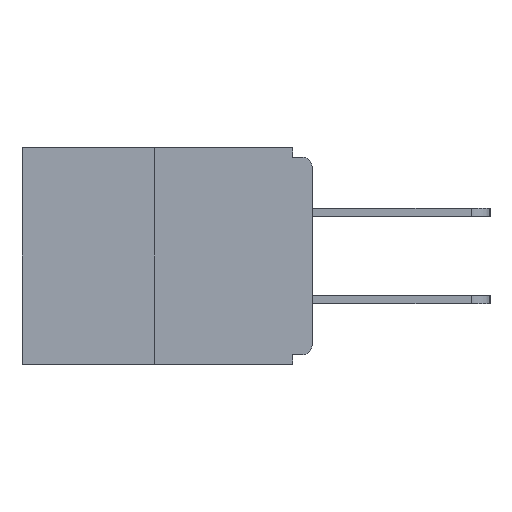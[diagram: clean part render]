
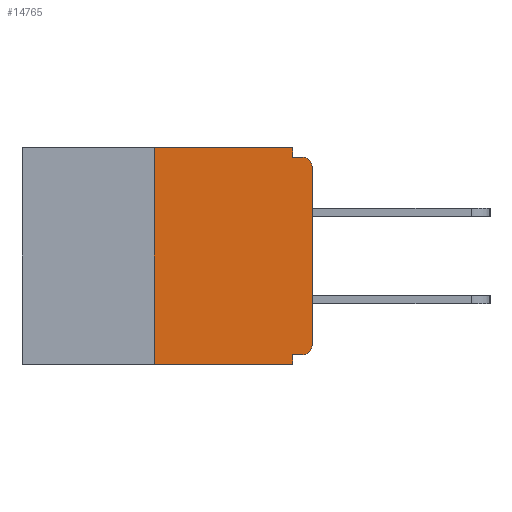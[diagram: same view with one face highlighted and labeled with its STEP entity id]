
A CAD part, left-side view. The second image highlights one B-rep face of the part: STEP entity #14765.
In plain terms, the highlighted planar face has unit normal (-1, 0, 0).
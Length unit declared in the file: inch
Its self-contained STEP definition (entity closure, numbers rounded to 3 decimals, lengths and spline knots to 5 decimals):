
#715 = DIRECTION ( 'NONE',  ( 0., 0., -1. ) ) ;
#1543 = CARTESIAN_POINT ( 'NONE',  ( 0., 0.015, -0.328 ) ) ;
#1964 = EDGE_CURVE ( 'NONE', #25171, #8974, #14584, .T. ) ;
#2256 = ORIENTED_EDGE ( 'NONE', *, *, #24477, .F. ) ;
#2329 = CARTESIAN_POINT ( 'NONE',  ( 0., 0.015, -0.03 ) ) ;
#2338 = VECTOR ( 'NONE', #20732, 39.37008 ) ;
#2395 = ORIENTED_EDGE ( 'NONE', *, *, #14337, .F. ) ;
#2488 = CARTESIAN_POINT ( 'NONE',  ( 0., 0.46, 0. ) ) ;
#2497 = VECTOR ( 'NONE', #12584, 39.37008 ) ;
#2853 = EDGE_CURVE ( 'NONE', #6195, #24756, #24557, .T. ) ;
#3083 = CIRCLE ( 'NONE', #25543, 0.015 ) ;
#3275 = ORIENTED_EDGE ( 'NONE', *, *, #10744, .T. ) ;
#3653 = VECTOR ( 'NONE', #22332, 39.37008 ) ;
#3779 = VECTOR ( 'NONE', #16435, 39.37008 ) ;
#3904 = DIRECTION ( 'NONE',  ( 0., 0., 1. ) ) ;
#4620 = CARTESIAN_POINT ( 'NONE',  ( 0., 0.031, -0.343 ) ) ;
#5089 = VECTOR ( 'NONE', #3904, 39.37008 ) ;
#6195 = VERTEX_POINT ( 'NONE', #13109 ) ;
#6420 = VERTEX_POINT ( 'NONE', #10481 ) ;
#6441 = ORIENTED_EDGE ( 'NONE', *, *, #17681, .T. ) ;
#6482 = LINE ( 'NONE', #14413, #2497 ) ;
#6577 = CARTESIAN_POINT ( 'NONE',  ( 0., 0., -0.328 ) ) ;
#7267 = DIRECTION ( 'NONE',  ( 0., -1., 0. ) ) ;
#7313 = ORIENTED_EDGE ( 'NONE', *, *, #8717, .F. ) ;
#7368 = VECTOR ( 'NONE', #715, 39.37008 ) ;
#7386 = VECTOR ( 'NONE', #23771, 39.37008 ) ;
#7506 = EDGE_LOOP ( 'NONE', ( #2256, #2395, #16970, #7572, #7313, #6441, #3275, #17072, #18509, #18242 ) ) ;
#7572 = ORIENTED_EDGE ( 'NONE', *, *, #2853, .F. ) ;
#8063 = PLANE ( 'NONE',  #14569 ) ;
#8174 = CARTESIAN_POINT ( 'NONE',  ( 0., 0., 0. ) ) ;
#8237 = CARTESIAN_POINT ( 'NONE',  ( 0., 0.015, -0.313 ) ) ;
#8386 = LINE ( 'NONE', #6577, #3653 ) ;
#8536 = EDGE_CURVE ( 'NONE', #12411, #24756, #15813, .T. ) ;
#8717 = EDGE_CURVE ( 'NONE', #11268, #6195, #8386, .T. ) ;
#8889 = VERTEX_POINT ( 'NONE', #10853 ) ;
#8974 = VERTEX_POINT ( 'NONE', #17737 ) ;
#9231 = LINE ( 'NONE', #19259, #21416 ) ;
#9463 = AXIS2_PLACEMENT_3D ( 'NONE', #2329, #22397, #22781 ) ;
#10149 = DIRECTION ( 'NONE',  ( 0., 0., -1. ) ) ;
#10419 = DIRECTION ( 'NONE',  ( 1., 0., 0. ) ) ;
#10436 = VERTEX_POINT ( 'NONE', #18286 ) ;
#10481 = CARTESIAN_POINT ( 'NONE',  ( 0., 0.031, 0. ) ) ;
#10744 = EDGE_CURVE ( 'NONE', #10436, #8889, #25646, .T. ) ;
#10853 = CARTESIAN_POINT ( 'NONE',  ( 0., 0., -0.03 ) ) ;
#11268 = VERTEX_POINT ( 'NONE', #1543 ) ;
#12109 = FACE_OUTER_BOUND ( 'NONE', #7506, .T. ) ;
#12255 = DIRECTION ( 'NONE',  ( 0., 0., -1. ) ) ;
#12411 = VERTEX_POINT ( 'NONE', #12732 ) ;
#12584 = DIRECTION ( 'NONE',  ( 0., 0., -1. ) ) ;
#12732 = CARTESIAN_POINT ( 'NONE',  ( 0., 0.25, -0.343 ) ) ;
#13109 = CARTESIAN_POINT ( 'NONE',  ( 0., 0.031, -0.328 ) ) ;
#14118 = EDGE_CURVE ( 'NONE', #6420, #25171, #6482, .T. ) ;
#14211 = DIRECTION ( 'NONE',  ( -1., 0., 0. ) ) ;
#14217 = CARTESIAN_POINT ( 'NONE',  ( 0., 0.25, 0. ) ) ;
#14337 = EDGE_CURVE ( 'NONE', #12411, #14476, #16310, .T. ) ;
#14413 = CARTESIAN_POINT ( 'NONE',  ( 0., 0.031, 0. ) ) ;
#14476 = VERTEX_POINT ( 'NONE', #15007 ) ;
#14569 = AXIS2_PLACEMENT_3D ( 'NONE', #2488, #10419, #10149 ) ;
#14584 = LINE ( 'NONE', #24496, #2338 ) ;
#14765 = ADVANCED_FACE ( 'NONE', ( #12109 ), #8063, .F. ) ;
#15007 = CARTESIAN_POINT ( 'NONE',  ( 0., 0.25, 0. ) ) ;
#15446 = CARTESIAN_POINT ( 'NONE',  ( 0., 0.46, -0.343 ) ) ;
#15813 = LINE ( 'NONE', #15446, #7386 ) ;
#16310 = LINE ( 'NONE', #14217, #3779 ) ;
#16435 = DIRECTION ( 'NONE',  ( 0., 0., 1. ) ) ;
#16731 = EDGE_CURVE ( 'NONE', #8889, #8974, #17353, .T. ) ;
#16970 = ORIENTED_EDGE ( 'NONE', *, *, #8536, .T. ) ;
#17072 = ORIENTED_EDGE ( 'NONE', *, *, #16731, .T. ) ;
#17353 = CIRCLE ( 'NONE', #9463, 0.015 ) ;
#17681 = EDGE_CURVE ( 'NONE', #11268, #10436, #3083, .T. ) ;
#17737 = CARTESIAN_POINT ( 'NONE',  ( 0., 0.015, -0.015 ) ) ;
#18242 = ORIENTED_EDGE ( 'NONE', *, *, #14118, .F. ) ;
#18286 = CARTESIAN_POINT ( 'NONE',  ( 0., 0., -0.313 ) ) ;
#18509 = ORIENTED_EDGE ( 'NONE', *, *, #1964, .F. ) ;
#19259 = CARTESIAN_POINT ( 'NONE',  ( 0., 0.46, 0. ) ) ;
#20271 = CARTESIAN_POINT ( 'NONE',  ( 0., 0.031, -0.343 ) ) ;
#20732 = DIRECTION ( 'NONE',  ( 0., -1., 0. ) ) ;
#21416 = VECTOR ( 'NONE', #7267, 39.37008 ) ;
#22332 = DIRECTION ( 'NONE',  ( 0., 1., 0. ) ) ;
#22397 = DIRECTION ( 'NONE',  ( -1., 0., 0. ) ) ;
#22781 = DIRECTION ( 'NONE',  ( 0., 0., -1. ) ) ;
#23771 = DIRECTION ( 'NONE',  ( 0., -1., 0. ) ) ;
#24477 = EDGE_CURVE ( 'NONE', #14476, #6420, #9231, .T. ) ;
#24496 = CARTESIAN_POINT ( 'NONE',  ( 0., 0., -0.015 ) ) ;
#24557 = LINE ( 'NONE', #20271, #7368 ) ;
#24756 = VERTEX_POINT ( 'NONE', #4620 ) ;
#25025 = CARTESIAN_POINT ( 'NONE',  ( 0., 0.031, -0.015 ) ) ;
#25171 = VERTEX_POINT ( 'NONE', #25025 ) ;
#25543 = AXIS2_PLACEMENT_3D ( 'NONE', #8237, #14211, #12255 ) ;
#25646 = LINE ( 'NONE', #8174, #5089 ) ;
